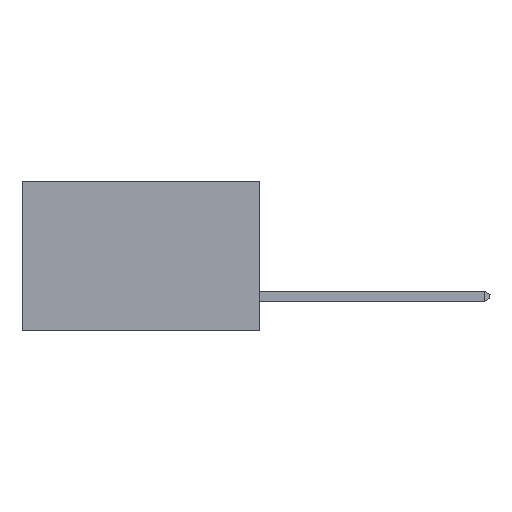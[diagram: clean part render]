
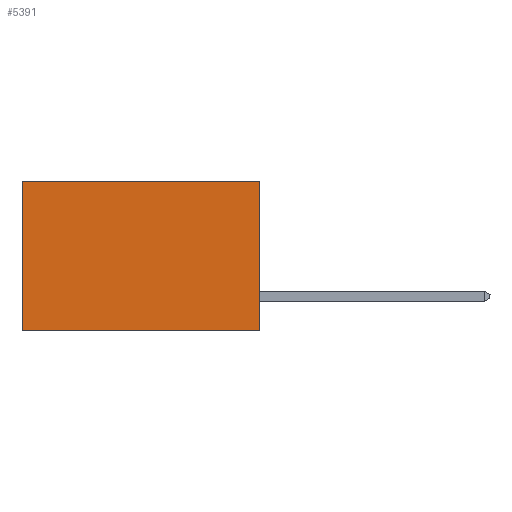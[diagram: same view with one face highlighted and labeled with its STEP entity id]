
A CAD part, left-side view. The second image highlights one B-rep face of the part: STEP entity #5391.
In plain terms, the highlighted planar face has unit normal (-1, 0, 0).
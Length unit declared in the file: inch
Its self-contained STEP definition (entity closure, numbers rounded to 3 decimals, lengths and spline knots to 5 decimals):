
#490 = LINE ( 'NONE', #6162, #8431 ) ;
#504 = VECTOR ( 'NONE', #2934, 39.37008 ) ;
#771 = CARTESIAN_POINT ( 'NONE',  ( 0.277, 0., 0. ) ) ;
#2045 = CARTESIAN_POINT ( 'NONE',  ( 0.277, 0., -0.37 ) ) ;
#2064 = VECTOR ( 'NONE', #5801, 39.37008 ) ;
#2383 = ORIENTED_EDGE ( 'NONE', *, *, #3891, .F. ) ;
#2792 = CARTESIAN_POINT ( 'NONE',  ( 0.277, 0.59, -0.37 ) ) ;
#2934 = DIRECTION ( 'NONE',  ( 0., 1., 0. ) ) ;
#2999 = EDGE_CURVE ( 'NONE', #8745, #5726, #5174, .T. ) ;
#3035 = VECTOR ( 'NONE', #6589, 39.37008 ) ;
#3458 = EDGE_CURVE ( 'NONE', #6797, #4697, #7035, .T. ) ;
#3891 = EDGE_CURVE ( 'NONE', #8745, #6797, #490, .T. ) ;
#4208 = CARTESIAN_POINT ( 'NONE',  ( 0.277, 0., -0.37 ) ) ;
#4531 = CARTESIAN_POINT ( 'NONE',  ( 0.277, 0.59, 0. ) ) ;
#4697 = VERTEX_POINT ( 'NONE', #2792 ) ;
#4753 = FACE_OUTER_BOUND ( 'NONE', #7660, .T. ) ;
#4832 = CARTESIAN_POINT ( 'NONE',  ( 0.277, 0., 0. ) ) ;
#5174 = LINE ( 'NONE', #4832, #3035 ) ;
#5300 = ORIENTED_EDGE ( 'NONE', *, *, #3458, .F. ) ;
#5391 = ADVANCED_FACE ( 'NONE', ( #4753 ), #6183, .F. ) ;
#5436 = EDGE_CURVE ( 'NONE', #5726, #4697, #6436, .T. ) ;
#5726 = VERTEX_POINT ( 'NONE', #4531 ) ;
#5801 = DIRECTION ( 'NONE',  ( 0., 0., -1. ) ) ;
#5815 = CARTESIAN_POINT ( 'NONE',  ( 0.277, 0.59, -0.37 ) ) ;
#5963 = DIRECTION ( 'NONE',  ( 0., 0., -1. ) ) ;
#6106 = DIRECTION ( 'NONE',  ( 0., 0., -1. ) ) ;
#6119 = DIRECTION ( 'NONE',  ( 1., 0., 0. ) ) ;
#6129 = CARTESIAN_POINT ( 'NONE',  ( 0.277, 0., -0.37 ) ) ;
#6162 = CARTESIAN_POINT ( 'NONE',  ( 0.277, 0., -0.37 ) ) ;
#6167 = AXIS2_PLACEMENT_3D ( 'NONE', #6129, #6119, #6106 ) ;
#6183 = PLANE ( 'NONE',  #6167 ) ;
#6436 = LINE ( 'NONE', #5815, #2064 ) ;
#6589 = DIRECTION ( 'NONE',  ( 0., 1., 0. ) ) ;
#6797 = VERTEX_POINT ( 'NONE', #4208 ) ;
#7035 = LINE ( 'NONE', #2045, #504 ) ;
#7536 = ORIENTED_EDGE ( 'NONE', *, *, #2999, .T. ) ;
#7660 = EDGE_LOOP ( 'NONE', ( #8022, #5300, #2383, #7536 ) ) ;
#8022 = ORIENTED_EDGE ( 'NONE', *, *, #5436, .T. ) ;
#8431 = VECTOR ( 'NONE', #5963, 39.37008 ) ;
#8745 = VERTEX_POINT ( 'NONE', #771 ) ;
